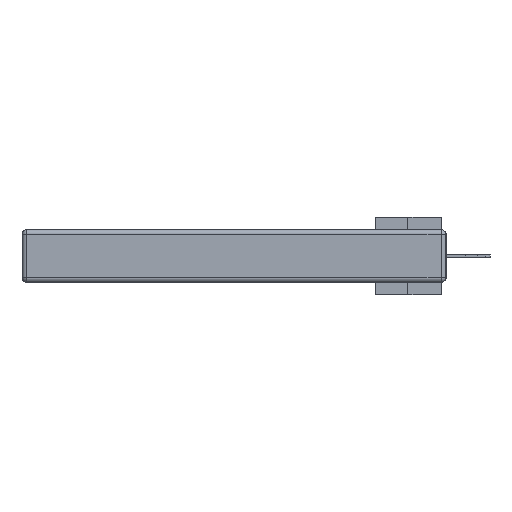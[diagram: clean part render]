
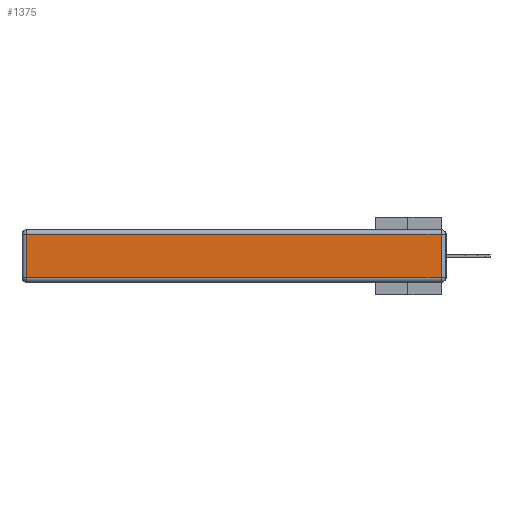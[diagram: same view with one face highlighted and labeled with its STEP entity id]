
A CAD part, left-side view. The second image highlights one B-rep face of the part: STEP entity #1375.
In plain terms, the highlighted planar face has unit normal (-1, 0, 0).
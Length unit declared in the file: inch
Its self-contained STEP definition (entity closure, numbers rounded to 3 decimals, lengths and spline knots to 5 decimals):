
#1375 = ADVANCED_FACE ( 'NONE', ( #19422 ), #5776, .T. ) ;
#1719 = LINE ( 'NONE', #33797, #8019 ) ;
#1794 = EDGE_LOOP ( 'NONE', ( #13581, #27392, #24915, #23086 ) ) ;
#1897 = AXIS2_PLACEMENT_3D ( 'NONE', #18511, #4191, #23190 ) ;
#3428 = VERTEX_POINT ( 'NONE', #15625 ) ;
#4191 = DIRECTION ( 'NONE',  ( -1., 0., 0. ) ) ;
#4624 = CARTESIAN_POINT ( 'NONE',  ( 0., 0.03, -0.343 ) ) ;
#5776 = PLANE ( 'NONE',  #1897 ) ;
#7077 = EDGE_CURVE ( 'NONE', #24926, #24285, #17053, .T. ) ;
#8019 = VECTOR ( 'NONE', #28768, 39.37008 ) ;
#8692 = VECTOR ( 'NONE', #20595, 39.37008 ) ;
#9062 = DIRECTION ( 'NONE',  ( 0., -1., 0. ) ) ;
#9462 = EDGE_CURVE ( 'NONE', #3428, #13227, #31466, .T. ) ;
#9508 = CARTESIAN_POINT ( 'NONE',  ( 0., 2.75, -0.03 ) ) ;
#9534 = LINE ( 'NONE', #4624, #8692 ) ;
#12318 = VECTOR ( 'NONE', #30460, 39.37008 ) ;
#13227 = VERTEX_POINT ( 'NONE', #27493 ) ;
#13581 = ORIENTED_EDGE ( 'NONE', *, *, #7077, .T. ) ;
#14412 = CARTESIAN_POINT ( 'NONE',  ( 0., 0.03, -0.313 ) ) ;
#15625 = CARTESIAN_POINT ( 'NONE',  ( 0., 0.03, -0.03 ) ) ;
#16132 = EDGE_CURVE ( 'NONE', #24285, #3428, #9534, .T. ) ;
#16200 = VECTOR ( 'NONE', #9062, 39.37008 ) ;
#17053 = LINE ( 'NONE', #30036, #16200 ) ;
#18511 = CARTESIAN_POINT ( 'NONE',  ( 0., 0., -0.343 ) ) ;
#19422 = FACE_OUTER_BOUND ( 'NONE', #1794, .T. ) ;
#20595 = DIRECTION ( 'NONE',  ( 0., 0., 1. ) ) ;
#23086 = ORIENTED_EDGE ( 'NONE', *, *, #32921, .T. ) ;
#23190 = DIRECTION ( 'NONE',  ( 0., 0., 1. ) ) ;
#24285 = VERTEX_POINT ( 'NONE', #14412 ) ;
#24866 = CARTESIAN_POINT ( 'NONE',  ( 0., 2.72, -0.313 ) ) ;
#24915 = ORIENTED_EDGE ( 'NONE', *, *, #9462, .T. ) ;
#24926 = VERTEX_POINT ( 'NONE', #24866 ) ;
#27392 = ORIENTED_EDGE ( 'NONE', *, *, #16132, .T. ) ;
#27493 = CARTESIAN_POINT ( 'NONE',  ( 0., 2.72, -0.03 ) ) ;
#28768 = DIRECTION ( 'NONE',  ( 0., 0., -1. ) ) ;
#30036 = CARTESIAN_POINT ( 'NONE',  ( 0., 0., -0.313 ) ) ;
#30460 = DIRECTION ( 'NONE',  ( 0., 1., 0. ) ) ;
#31466 = LINE ( 'NONE', #9508, #12318 ) ;
#32921 = EDGE_CURVE ( 'NONE', #13227, #24926, #1719, .T. ) ;
#33797 = CARTESIAN_POINT ( 'NONE',  ( 0., 2.72, -0.343 ) ) ;
